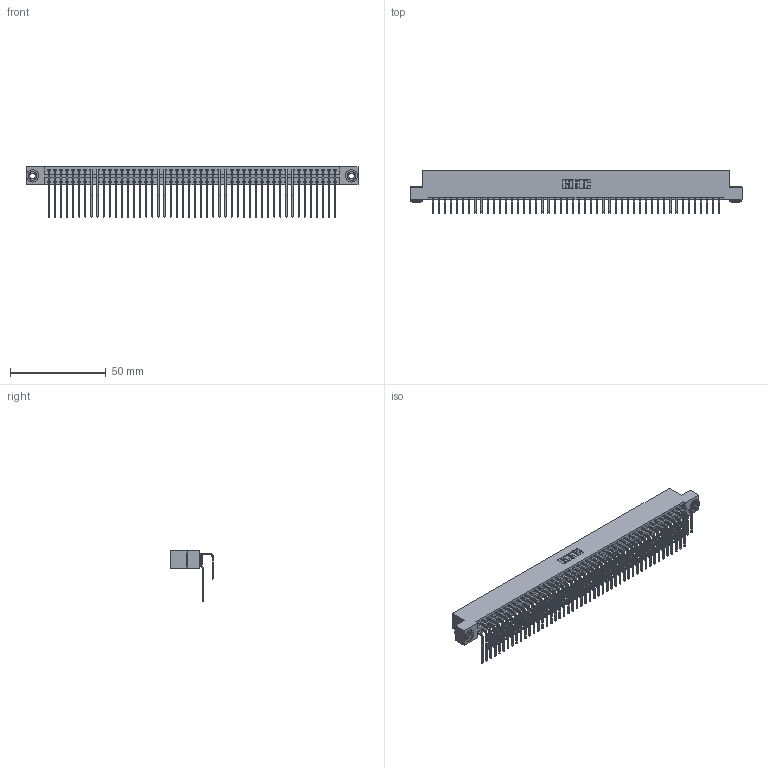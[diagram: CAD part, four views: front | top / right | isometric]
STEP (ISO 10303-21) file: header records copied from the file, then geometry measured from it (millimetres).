
FILE_DESCRIPTION (( 'STEP AP203' ), '1' );
FILE_NAME ('346-096-558-203.STEP', '2022-05-26T16:59:56', ( '' ), ( '' ), 'SwSTEP 2.0', 'SolidWorks 2020', '' );
FILE_SCHEMA (( 'CONFIG_CONTROL_DESIGN' ));
Length unit declared in the file: inch
Products named in the file (5): 345-292-001_558 559 Tail - 1; 345-292-001_558 Tail - 2; 346 Part_Flush Mounting Lugs - 0.156 Dia-TH; 346-096-558-203; 345-250-002_345-250-002-102
Assembly tree (99 placements, depth 2):
  346-096-558-203
    346 Part_Flush Mounting Lugs - 0.156 Dia-TH
    345-292-001_558 559 Tail - 1  x48
    345-292-001_558 Tail - 2  x48
    345-250-002_345-250-002-102  x2
Bounding box: 172.97 x 22.16 x 26.16 mm (x, y, z)
Volume: 17468.8 mm3; surface area: 27011.9 mm2
Topology: 99 solids, 99 shells, 5358 faces, 15897 edges, 10466 vertices
Faces by surface type: plane 3652, cylinder 1698, cone 8
Entity records: 33368 total; most frequent: CARTESIAN_POINT 5524, ORIENTED_EDGE 5398, DIRECTION 4921, EDGE_CURVE 2699, LINE 2311, VECTOR 2311, VERTEX_POINT 1794, AXIS2_PLACEMENT_3D 1305
